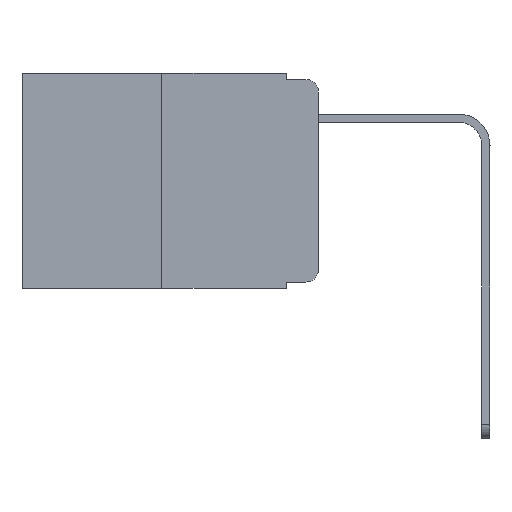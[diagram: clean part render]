
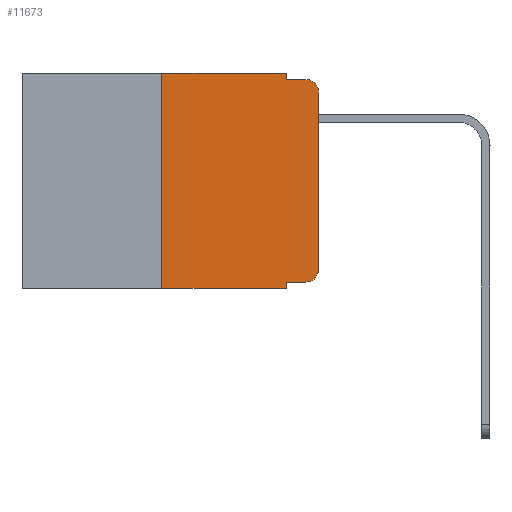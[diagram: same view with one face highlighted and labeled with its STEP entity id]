
A CAD part, left-side view. The second image highlights one B-rep face of the part: STEP entity #11673.
In plain terms, the highlighted planar face has unit normal (-1, 0, 0).
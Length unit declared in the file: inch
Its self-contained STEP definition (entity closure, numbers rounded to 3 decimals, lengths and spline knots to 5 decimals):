
#36 = EDGE_CURVE ( 'NONE', #4284, #4712, #8886, .T. ) ;
#128 = VECTOR ( 'NONE', #6160, 39.37008 ) ;
#151 = ORIENTED_EDGE ( 'NONE', *, *, #12595, .F. ) ;
#508 = DIRECTION ( 'NONE',  ( 0., 0., -1. ) ) ;
#860 = EDGE_CURVE ( 'NONE', #9202, #4549, #10804, .T. ) ;
#991 = CARTESIAN_POINT ( 'NONE',  ( 0., 0.25, 0. ) ) ;
#1109 = DIRECTION ( 'NONE',  ( 0., -1., 0. ) ) ;
#1183 = ORIENTED_EDGE ( 'NONE', *, *, #11804, .F. ) ;
#1395 = LINE ( 'NONE', #5428, #9478 ) ;
#1697 = LINE ( 'NONE', #12910, #12365 ) ;
#2438 = PLANE ( 'NONE',  #5101 ) ;
#2568 = VECTOR ( 'NONE', #7337, 39.37008 ) ;
#2604 = CARTESIAN_POINT ( 'NONE',  ( 0., 0.051, -0.01 ) ) ;
#2758 = ORIENTED_EDGE ( 'NONE', *, *, #9053, .F. ) ;
#3413 = CARTESIAN_POINT ( 'NONE',  ( 0., 0.473, -0.343 ) ) ;
#3530 = DIRECTION ( 'NONE',  ( 0., 0., -1. ) ) ;
#4284 = VERTEX_POINT ( 'NONE', #11992 ) ;
#4324 = FACE_OUTER_BOUND ( 'NONE', #13367, .T. ) ;
#4433 = CARTESIAN_POINT ( 'NONE',  ( 0., 0., -0.313 ) ) ;
#4489 = DIRECTION ( 'NONE',  ( 0., -1., 0. ) ) ;
#4549 = VERTEX_POINT ( 'NONE', #5921 ) ;
#4712 = VERTEX_POINT ( 'NONE', #9439 ) ;
#4927 = CARTESIAN_POINT ( 'NONE',  ( 0., 0., 0. ) ) ;
#5035 = VECTOR ( 'NONE', #7043, 39.37008 ) ;
#5101 = AXIS2_PLACEMENT_3D ( 'NONE', #6641, #12812, #10730 ) ;
#5118 = CIRCLE ( 'NONE', #7225, 0.02 ) ;
#5185 = AXIS2_PLACEMENT_3D ( 'NONE', #7853, #5820, #8809 ) ;
#5399 = DIRECTION ( 'NONE',  ( 0., 0., 1. ) ) ;
#5428 = CARTESIAN_POINT ( 'NONE',  ( 0., 0.051, -0.333 ) ) ;
#5523 = CARTESIAN_POINT ( 'NONE',  ( 0., 0.25, 0. ) ) ;
#5635 = VECTOR ( 'NONE', #5399, 39.37008 ) ;
#5706 = CARTESIAN_POINT ( 'NONE',  ( 0., 0.051, 0. ) ) ;
#5771 = ORIENTED_EDGE ( 'NONE', *, *, #6099, .T. ) ;
#5820 = DIRECTION ( 'NONE',  ( -1., 0., 0. ) ) ;
#5921 = CARTESIAN_POINT ( 'NONE',  ( 0., 0.02, -0.01 ) ) ;
#5966 = LINE ( 'NONE', #5706, #11419 ) ;
#6064 = EDGE_CURVE ( 'NONE', #12128, #9202, #1697, .T. ) ;
#6099 = EDGE_CURVE ( 'NONE', #11265, #4549, #5118, .T. ) ;
#6160 = DIRECTION ( 'NONE',  ( 0., -1., 0. ) ) ;
#6285 = VERTEX_POINT ( 'NONE', #9056 ) ;
#6340 = CARTESIAN_POINT ( 'NONE',  ( 0., 0.051, -0.01 ) ) ;
#6641 = CARTESIAN_POINT ( 'NONE',  ( 0., 0.473, 0. ) ) ;
#7005 = ORIENTED_EDGE ( 'NONE', *, *, #36, .T. ) ;
#7043 = DIRECTION ( 'NONE',  ( 0., -1., 0. ) ) ;
#7225 = AXIS2_PLACEMENT_3D ( 'NONE', #7895, #8910, #12323 ) ;
#7337 = DIRECTION ( 'NONE',  ( 0., 0., 1. ) ) ;
#7853 = CARTESIAN_POINT ( 'NONE',  ( 0., 0.02, -0.313 ) ) ;
#7895 = CARTESIAN_POINT ( 'NONE',  ( 0., 0.02, -0.03 ) ) ;
#8369 = ORIENTED_EDGE ( 'NONE', *, *, #6064, .F. ) ;
#8394 = LINE ( 'NONE', #4927, #2568 ) ;
#8499 = EDGE_CURVE ( 'NONE', #8683, #11265, #8394, .T. ) ;
#8683 = VERTEX_POINT ( 'NONE', #4433 ) ;
#8809 = DIRECTION ( 'NONE',  ( 0., 0., -1. ) ) ;
#8886 = LINE ( 'NONE', #3413, #5035 ) ;
#8910 = DIRECTION ( 'NONE',  ( -1., 0., 0. ) ) ;
#9009 = LINE ( 'NONE', #991, #5635 ) ;
#9053 = EDGE_CURVE ( 'NONE', #11714, #12128, #10495, .T. ) ;
#9056 = CARTESIAN_POINT ( 'NONE',  ( 0., 0.051, -0.333 ) ) ;
#9095 = ORIENTED_EDGE ( 'NONE', *, *, #11564, .T. ) ;
#9202 = VERTEX_POINT ( 'NONE', #6340 ) ;
#9239 = CARTESIAN_POINT ( 'NONE',  ( 0., 0.473, 0. ) ) ;
#9276 = CARTESIAN_POINT ( 'NONE',  ( 0., 0.051, 0. ) ) ;
#9439 = CARTESIAN_POINT ( 'NONE',  ( 0., 0.051, -0.343 ) ) ;
#9478 = VECTOR ( 'NONE', #1109, 39.37008 ) ;
#10221 = CARTESIAN_POINT ( 'NONE',  ( 0., 0.02, -0.333 ) ) ;
#10495 = LINE ( 'NONE', #9239, #128 ) ;
#10730 = DIRECTION ( 'NONE',  ( 0., 0., -1. ) ) ;
#10741 = VECTOR ( 'NONE', #4489, 39.37008 ) ;
#10804 = LINE ( 'NONE', #2604, #10741 ) ;
#11091 = EDGE_CURVE ( 'NONE', #13067, #8683, #12399, .T. ) ;
#11265 = VERTEX_POINT ( 'NONE', #12203 ) ;
#11419 = VECTOR ( 'NONE', #508, 39.37008 ) ;
#11564 = EDGE_CURVE ( 'NONE', #6285, #13067, #1395, .T. ) ;
#11673 = ADVANCED_FACE ( 'NONE', ( #4324 ), #2438, .F. ) ;
#11714 = VERTEX_POINT ( 'NONE', #5523 ) ;
#11804 = EDGE_CURVE ( 'NONE', #6285, #4712, #5966, .T. ) ;
#11915 = ORIENTED_EDGE ( 'NONE', *, *, #8499, .T. ) ;
#11992 = CARTESIAN_POINT ( 'NONE',  ( 0., 0.25, -0.343 ) ) ;
#12128 = VERTEX_POINT ( 'NONE', #9276 ) ;
#12203 = CARTESIAN_POINT ( 'NONE',  ( 0., 0., -0.03 ) ) ;
#12323 = DIRECTION ( 'NONE',  ( 0., 0., -1. ) ) ;
#12365 = VECTOR ( 'NONE', #3530, 39.37008 ) ;
#12399 = CIRCLE ( 'NONE', #5185, 0.02 ) ;
#12595 = EDGE_CURVE ( 'NONE', #4284, #11714, #9009, .T. ) ;
#12786 = ORIENTED_EDGE ( 'NONE', *, *, #11091, .T. ) ;
#12812 = DIRECTION ( 'NONE',  ( 1., 0., 0. ) ) ;
#12910 = CARTESIAN_POINT ( 'NONE',  ( 0., 0.051, 0. ) ) ;
#13023 = ORIENTED_EDGE ( 'NONE', *, *, #860, .F. ) ;
#13067 = VERTEX_POINT ( 'NONE', #10221 ) ;
#13367 = EDGE_LOOP ( 'NONE', ( #11915, #5771, #13023, #8369, #2758, #151, #7005, #1183, #9095, #12786 ) ) ;
